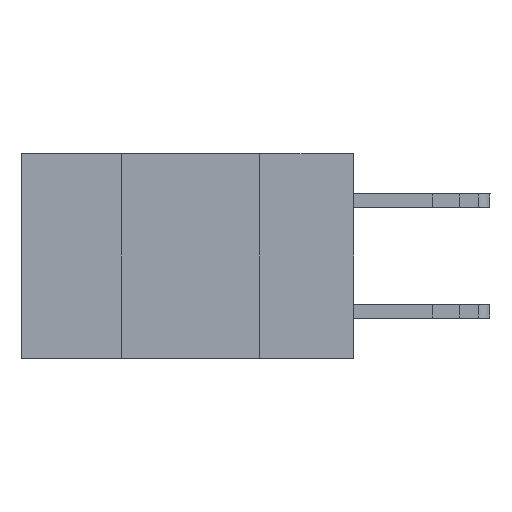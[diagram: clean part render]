
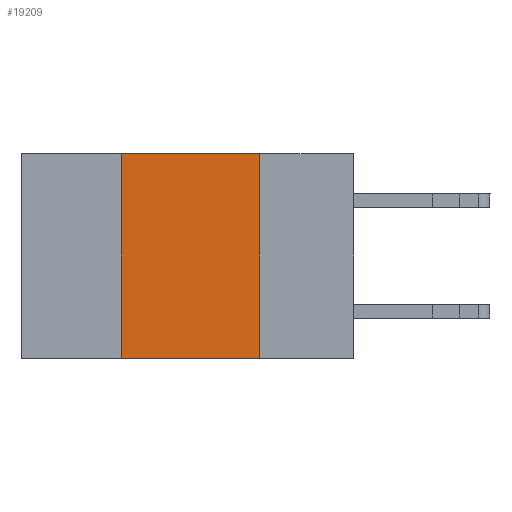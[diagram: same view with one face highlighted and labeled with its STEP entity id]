
A CAD part, left-side view. The second image highlights one B-rep face of the part: STEP entity #19209.
In plain terms, the highlighted planar face has unit normal (-1, 0, 0).
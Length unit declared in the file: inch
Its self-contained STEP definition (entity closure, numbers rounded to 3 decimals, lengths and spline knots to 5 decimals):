
#125 = ORIENTED_EDGE ( 'NONE', *, *, #16141, .F. ) ;
#392 = VECTOR ( 'NONE', #22111, 39.37008 ) ;
#906 = LINE ( 'NONE', #27018, #21250 ) ;
#2138 = ORIENTED_EDGE ( 'NONE', *, *, #12007, .F. ) ;
#2499 = EDGE_LOOP ( 'NONE', ( #29904, #125, #2138, #19987 ) ) ;
#3689 = LINE ( 'NONE', #20093, #392 ) ;
#5814 = LINE ( 'NONE', #22530, #30795 ) ;
#7323 = FACE_OUTER_BOUND ( 'NONE', #2499, .T. ) ;
#7406 = AXIS2_PLACEMENT_3D ( 'NONE', #19321, #28883, #14655 ) ;
#7720 = CARTESIAN_POINT ( 'NONE',  ( 0., 0.17, 0. ) ) ;
#9799 = PLANE ( 'NONE',  #7406 ) ;
#11554 = EDGE_CURVE ( 'NONE', #18733, #21880, #906, .T. ) ;
#12007 = EDGE_CURVE ( 'NONE', #18733, #16127, #3689, .T. ) ;
#12452 = EDGE_CURVE ( 'NONE', #22415, #21880, #19587, .T. ) ;
#12825 = CARTESIAN_POINT ( 'NONE',  ( 0., 0.17, -0.37 ) ) ;
#14521 = CARTESIAN_POINT ( 'NONE',  ( 0., 0.17, 0. ) ) ;
#14655 = DIRECTION ( 'NONE',  ( 0., 0., -1. ) ) ;
#16127 = VERTEX_POINT ( 'NONE', #17999 ) ;
#16141 = EDGE_CURVE ( 'NONE', #16127, #22415, #5814, .T. ) ;
#16467 = CARTESIAN_POINT ( 'NONE',  ( 0., 0.42, -0.37 ) ) ;
#17999 = CARTESIAN_POINT ( 'NONE',  ( 0., 0.42, 0. ) ) ;
#18733 = VERTEX_POINT ( 'NONE', #16467 ) ;
#19209 = ADVANCED_FACE ( 'NONE', ( #7323 ), #9799, .F. ) ;
#19321 = CARTESIAN_POINT ( 'NONE',  ( 0., 0.6, 0. ) ) ;
#19580 = VECTOR ( 'NONE', #27108, 39.37008 ) ;
#19587 = LINE ( 'NONE', #7720, #19580 ) ;
#19973 = DIRECTION ( 'NONE',  ( 0., -1., 0. ) ) ;
#19987 = ORIENTED_EDGE ( 'NONE', *, *, #11554, .T. ) ;
#20093 = CARTESIAN_POINT ( 'NONE',  ( 0., 0.42, 0. ) ) ;
#20337 = DIRECTION ( 'NONE',  ( 0., -1., 0. ) ) ;
#21250 = VECTOR ( 'NONE', #19973, 39.37008 ) ;
#21880 = VERTEX_POINT ( 'NONE', #12825 ) ;
#22111 = DIRECTION ( 'NONE',  ( 0., 0., 1. ) ) ;
#22415 = VERTEX_POINT ( 'NONE', #14521 ) ;
#22530 = CARTESIAN_POINT ( 'NONE',  ( 0., 0.6, 0. ) ) ;
#27018 = CARTESIAN_POINT ( 'NONE',  ( 0., 0.6, -0.37 ) ) ;
#27108 = DIRECTION ( 'NONE',  ( 0., 0., -1. ) ) ;
#28883 = DIRECTION ( 'NONE',  ( 1., 0., 0. ) ) ;
#29904 = ORIENTED_EDGE ( 'NONE', *, *, #12452, .F. ) ;
#30795 = VECTOR ( 'NONE', #20337, 39.37008 ) ;
